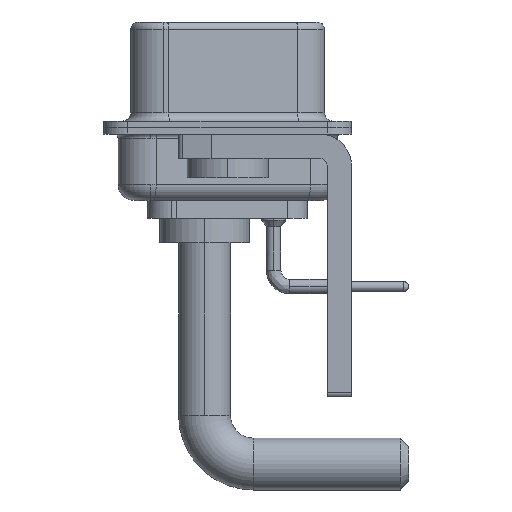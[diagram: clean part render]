
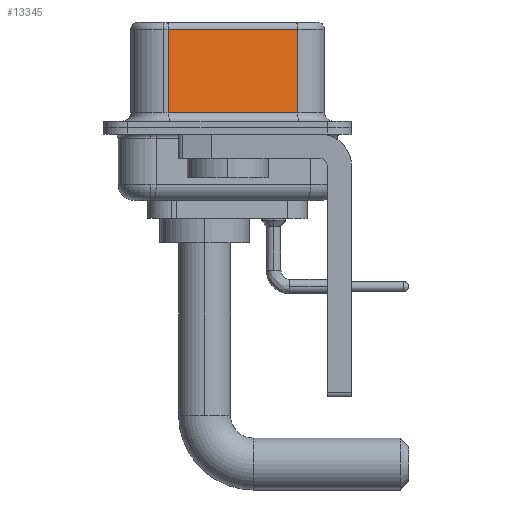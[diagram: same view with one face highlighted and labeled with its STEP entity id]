
A CAD part, left-side view. The second image highlights one B-rep face of the part: STEP entity #13345.
In plain terms, the highlighted planar face has unit normal (-0.985, -0.174, 0).
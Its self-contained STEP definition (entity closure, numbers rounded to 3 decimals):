
#429 = VERTEX_POINT ( 'NONE', #11308 ) ;
#2478 = VERTEX_POINT ( 'NONE', #2998 ) ;
#2998 = CARTESIAN_POINT ( 'NONE',  ( 5.132, -4.322, 0.9 ) ) ;
#3087 = CARTESIAN_POINT ( 'NONE',  ( 5.132, -4.322, 6.52 ) ) ;
#3279 = DIRECTION ( 'NONE',  ( 0., 0., -1. ) ) ;
#3422 = CARTESIAN_POINT ( 'NONE',  ( 3.73, 3.628, 0.9 ) ) ;
#3484 = CARTESIAN_POINT ( 'NONE',  ( 3.73, 3.628, 6.52 ) ) ;
#3693 = VERTEX_POINT ( 'NONE', #3422 ) ;
#4577 = EDGE_CURVE ( 'NONE', #429, #3693, #22344, .T. ) ;
#5104 = DIRECTION ( 'NONE',  ( 0.985, 0.174, 0. ) ) ;
#5229 = FACE_OUTER_BOUND ( 'NONE', #9860, .T. ) ;
#5928 = LINE ( 'NONE', #7680, #10443 ) ;
#7680 = CARTESIAN_POINT ( 'NONE',  ( 5.132, -4.322, 6.02 ) ) ;
#8929 = VERTEX_POINT ( 'NONE', #13559 ) ;
#9393 = ORIENTED_EDGE ( 'NONE', *, *, #4577, .T. ) ;
#9860 = EDGE_LOOP ( 'NONE', ( #17283, #21371, #9393, #23799 ) ) ;
#10443 = VECTOR ( 'NONE', #15563, 1000. ) ;
#10736 = DIRECTION ( 'NONE',  ( -0.174, 0.985, 0. ) ) ;
#10924 = CARTESIAN_POINT ( 'NONE',  ( 5.132, -4.322, 6.52 ) ) ;
#11308 = CARTESIAN_POINT ( 'NONE',  ( 3.73, 3.628, 6.02 ) ) ;
#13156 = LINE ( 'NONE', #10924, #15156 ) ;
#13345 = ADVANCED_FACE ( 'NONE', ( #5229 ), #20273, .F. ) ;
#13559 = CARTESIAN_POINT ( 'NONE',  ( 5.132, -4.322, 6.02 ) ) ;
#14328 = VECTOR ( 'NONE', #14777, 1000. ) ;
#14777 = DIRECTION ( 'NONE',  ( 0., 0., -1. ) ) ;
#15156 = VECTOR ( 'NONE', #3279, 1000. ) ;
#15563 = DIRECTION ( 'NONE',  ( -0.174, 0.985, 0. ) ) ;
#16059 = EDGE_CURVE ( 'NONE', #3693, #2478, #22425, .T. ) ;
#16076 = VECTOR ( 'NONE', #20402, 1000. ) ;
#17283 = ORIENTED_EDGE ( 'NONE', *, *, #20610, .F. ) ;
#20273 = PLANE ( 'NONE',  #23210 ) ;
#20402 = DIRECTION ( 'NONE',  ( 0.174, -0.985, 0. ) ) ;
#20610 = EDGE_CURVE ( 'NONE', #8929, #2478, #13156, .T. ) ;
#20644 = CARTESIAN_POINT ( 'NONE',  ( 5.132, -4.322, 0.9 ) ) ;
#21371 = ORIENTED_EDGE ( 'NONE', *, *, #24312, .T. ) ;
#22344 = LINE ( 'NONE', #3484, #14328 ) ;
#22425 = LINE ( 'NONE', #20644, #16076 ) ;
#23210 = AXIS2_PLACEMENT_3D ( 'NONE', #3087, #5104, #10736 ) ;
#23799 = ORIENTED_EDGE ( 'NONE', *, *, #16059, .T. ) ;
#24312 = EDGE_CURVE ( 'NONE', #8929, #429, #5928, .T. ) ;
